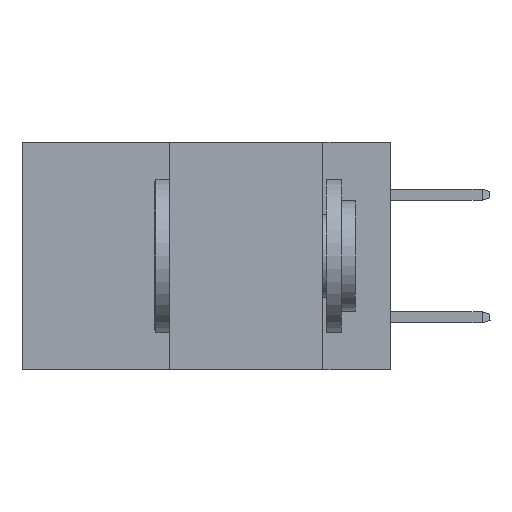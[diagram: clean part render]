
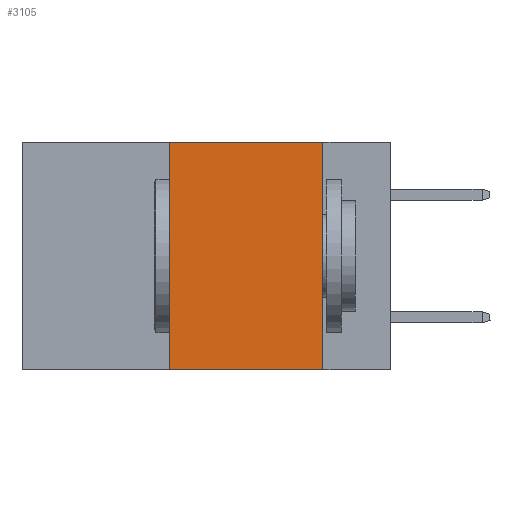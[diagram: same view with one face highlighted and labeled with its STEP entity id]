
A CAD part, left-side view. The second image highlights one B-rep face of the part: STEP entity #3105.
In plain terms, the highlighted planar face has unit normal (-1, 0, 0).
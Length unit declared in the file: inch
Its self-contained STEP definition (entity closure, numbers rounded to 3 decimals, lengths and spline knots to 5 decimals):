
#47 = DIRECTION ( 'NONE',  ( 0., 0., -1. ) ) ;
#64 = EDGE_CURVE ( 'NONE', #7807, #1318, #3741, .T. ) ;
#65 = DIRECTION ( 'NONE',  ( 1., 0., 0. ) ) ;
#66 = ORIENTED_EDGE ( 'NONE', *, *, #9154, .F. ) ;
#101 = CARTESIAN_POINT ( 'NONE',  ( 0., 0.11, 0. ) ) ;
#516 = LINE ( 'NONE', #2988, #8324 ) ;
#546 = ORIENTED_EDGE ( 'NONE', *, *, #7853, .F. ) ;
#1175 = EDGE_CURVE ( 'NONE', #3011, #1318, #516, .T. ) ;
#1318 = VERTEX_POINT ( 'NONE', #5916 ) ;
#1481 = DIRECTION ( 'NONE',  ( 0., 0., -1. ) ) ;
#1880 = ORIENTED_EDGE ( 'NONE', *, *, #64, .F. ) ;
#1989 = VECTOR ( 'NONE', #7699, 39.37008 ) ;
#2159 = CARTESIAN_POINT ( 'NONE',  ( 0., 0.36, -0.37 ) ) ;
#2236 = CARTESIAN_POINT ( 'NONE',  ( 0., 0.11, 0. ) ) ;
#2451 = DIRECTION ( 'NONE',  ( 0., 0., 1. ) ) ;
#2988 = CARTESIAN_POINT ( 'NONE',  ( 0., 0.6, -0.37 ) ) ;
#3011 = VERTEX_POINT ( 'NONE', #2159 ) ;
#3105 = ADVANCED_FACE ( 'NONE', ( #3948 ), #3681, .F. ) ;
#3681 = PLANE ( 'NONE',  #6057 ) ;
#3741 = LINE ( 'NONE', #2236, #7963 ) ;
#3948 = FACE_OUTER_BOUND ( 'NONE', #7949, .T. ) ;
#3983 = DIRECTION ( 'NONE',  ( 0., -1., 0. ) ) ;
#4000 = LINE ( 'NONE', #5440, #1989 ) ;
#4741 = CARTESIAN_POINT ( 'NONE',  ( 0., 0.36, 0. ) ) ;
#5440 = CARTESIAN_POINT ( 'NONE',  ( 0., 0.6, 0. ) ) ;
#5665 = LINE ( 'NONE', #4741, #9407 ) ;
#5916 = CARTESIAN_POINT ( 'NONE',  ( 0., 0.11, -0.37 ) ) ;
#6057 = AXIS2_PLACEMENT_3D ( 'NONE', #7185, #65, #47 ) ;
#6621 = ORIENTED_EDGE ( 'NONE', *, *, #1175, .T. ) ;
#7185 = CARTESIAN_POINT ( 'NONE',  ( 0., 0.6, 0. ) ) ;
#7699 = DIRECTION ( 'NONE',  ( 0., -1., 0. ) ) ;
#7807 = VERTEX_POINT ( 'NONE', #101 ) ;
#7853 = EDGE_CURVE ( 'NONE', #3011, #9701, #5665, .T. ) ;
#7949 = EDGE_LOOP ( 'NONE', ( #1880, #66, #546, #6621 ) ) ;
#7963 = VECTOR ( 'NONE', #1481, 39.37008 ) ;
#8324 = VECTOR ( 'NONE', #3983, 39.37008 ) ;
#9104 = CARTESIAN_POINT ( 'NONE',  ( 0., 0.36, 0. ) ) ;
#9154 = EDGE_CURVE ( 'NONE', #9701, #7807, #4000, .T. ) ;
#9407 = VECTOR ( 'NONE', #2451, 39.37008 ) ;
#9701 = VERTEX_POINT ( 'NONE', #9104 ) ;
